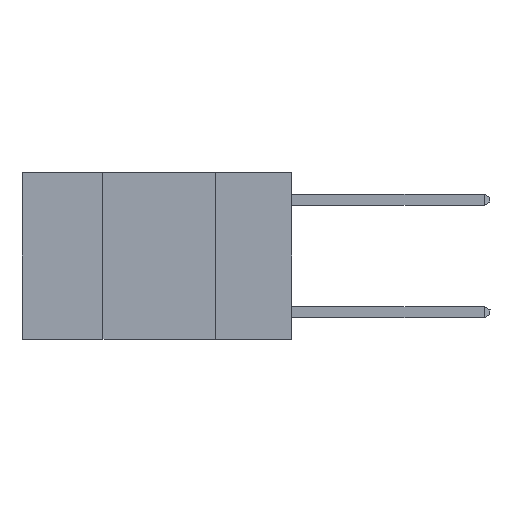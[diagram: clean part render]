
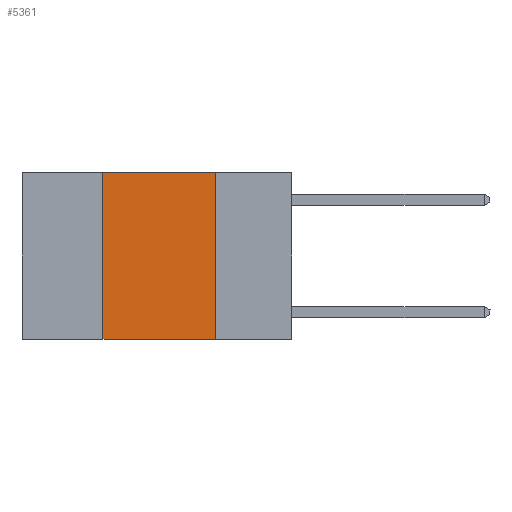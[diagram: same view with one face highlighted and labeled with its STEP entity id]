
A CAD part, left-side view. The second image highlights one B-rep face of the part: STEP entity #5361.
In plain terms, the highlighted planar face has unit normal (-1, 0, 0).
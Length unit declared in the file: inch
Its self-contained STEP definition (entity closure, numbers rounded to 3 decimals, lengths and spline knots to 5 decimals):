
#282 = ORIENTED_EDGE ( 'NONE', *, *, #1948, .F. ) ;
#372 = DIRECTION ( 'NONE',  ( 0., -1., 0. ) ) ;
#487 = ORIENTED_EDGE ( 'NONE', *, *, #8764, .F. ) ;
#503 = EDGE_CURVE ( 'NONE', #16436, #15555, #1392, .T. ) ;
#540 = ORIENTED_EDGE ( 'NONE', *, *, #8416, .F. ) ;
#791 = ORIENTED_EDGE ( 'NONE', *, *, #503, .T. ) ;
#1392 = LINE ( 'NONE', #13445, #12646 ) ;
#1399 = CARTESIAN_POINT ( 'NONE',  ( 0., 0.42, 0. ) ) ;
#1948 = EDGE_CURVE ( 'NONE', #16142, #15555, #2678, .T. ) ;
#2678 = LINE ( 'NONE', #4989, #10057 ) ;
#3696 = VERTEX_POINT ( 'NONE', #1399 ) ;
#4096 = VECTOR ( 'NONE', #6888, 39.37008 ) ;
#4190 = CARTESIAN_POINT ( 'NONE',  ( 0., 0.6, 0. ) ) ;
#4509 = CARTESIAN_POINT ( 'NONE',  ( 0., 0.6, 0. ) ) ;
#4989 = CARTESIAN_POINT ( 'NONE',  ( 0., 0.17, 0. ) ) ;
#5254 = CARTESIAN_POINT ( 'NONE',  ( 0., 0.17, -0.37 ) ) ;
#5361 = ADVANCED_FACE ( 'NONE', ( #11178 ), #13022, .F. ) ;
#5395 = CARTESIAN_POINT ( 'NONE',  ( 0., 0.42, 0. ) ) ;
#5717 = DIRECTION ( 'NONE',  ( 1., 0., 0. ) ) ;
#6032 = DIRECTION ( 'NONE',  ( 0., -1., 0. ) ) ;
#6888 = DIRECTION ( 'NONE',  ( 0., 0., 1. ) ) ;
#8086 = LINE ( 'NONE', #5395, #4096 ) ;
#8416 = EDGE_CURVE ( 'NONE', #16436, #3696, #8086, .T. ) ;
#8764 = EDGE_CURVE ( 'NONE', #3696, #16142, #10803, .T. ) ;
#9155 = CARTESIAN_POINT ( 'NONE',  ( 0., 0.17, 0. ) ) ;
#9280 = EDGE_LOOP ( 'NONE', ( #282, #487, #540, #791 ) ) ;
#9640 = CARTESIAN_POINT ( 'NONE',  ( 0., 0.42, -0.37 ) ) ;
#9867 = VECTOR ( 'NONE', #6032, 39.37008 ) ;
#10057 = VECTOR ( 'NONE', #15146, 39.37008 ) ;
#10803 = LINE ( 'NONE', #4509, #9867 ) ;
#11178 = FACE_OUTER_BOUND ( 'NONE', #9280, .T. ) ;
#12646 = VECTOR ( 'NONE', #372, 39.37008 ) ;
#13022 = PLANE ( 'NONE',  #15124 ) ;
#13445 = CARTESIAN_POINT ( 'NONE',  ( 0., 0.6, -0.37 ) ) ;
#15124 = AXIS2_PLACEMENT_3D ( 'NONE', #4190, #5717, #15841 ) ;
#15146 = DIRECTION ( 'NONE',  ( 0., 0., -1. ) ) ;
#15555 = VERTEX_POINT ( 'NONE', #5254 ) ;
#15841 = DIRECTION ( 'NONE',  ( 0., 0., -1. ) ) ;
#16142 = VERTEX_POINT ( 'NONE', #9155 ) ;
#16436 = VERTEX_POINT ( 'NONE', #9640 ) ;
